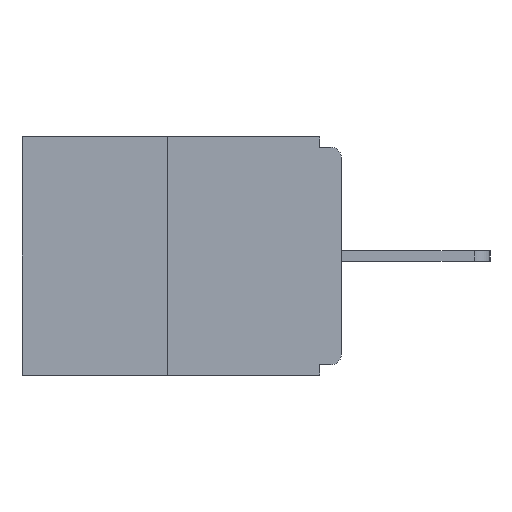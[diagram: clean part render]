
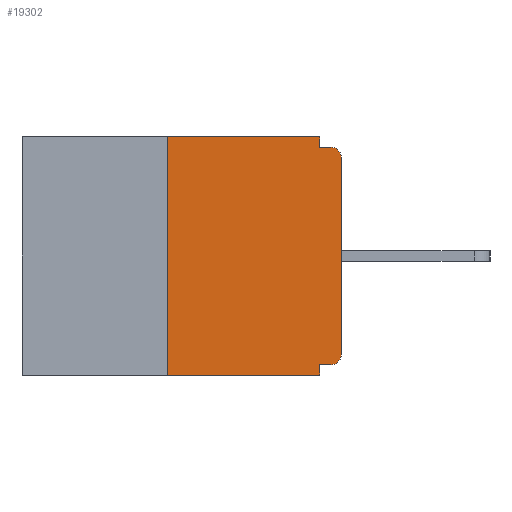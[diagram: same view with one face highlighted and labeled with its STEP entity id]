
A CAD part, left-side view. The second image highlights one B-rep face of the part: STEP entity #19302.
In plain terms, the highlighted planar face has unit normal (-1, 0, 0).
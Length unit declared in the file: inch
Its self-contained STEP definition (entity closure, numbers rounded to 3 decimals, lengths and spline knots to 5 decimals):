
#71 = CIRCLE ( 'NONE', #488, 0.015 ) ;
#295 = CIRCLE ( 'NONE', #757, 0.015 ) ;
#488 = AXIS2_PLACEMENT_3D ( 'NONE', #14695, #5281, #16189 ) ;
#510 = ORIENTED_EDGE ( 'NONE', *, *, #3146, .F. ) ;
#752 = LINE ( 'NONE', #2765, #15977 ) ;
#757 = AXIS2_PLACEMENT_3D ( 'NONE', #793, #11916, #2405 ) ;
#784 = VECTOR ( 'NONE', #14460, 39.37008 ) ;
#793 = CARTESIAN_POINT ( 'NONE',  ( 0., 0.015, -0.03 ) ) ;
#1218 = VERTEX_POINT ( 'NONE', #6164 ) ;
#1501 = CARTESIAN_POINT ( 'NONE',  ( 0., 0.031, 0. ) ) ;
#2095 = CARTESIAN_POINT ( 'NONE',  ( 0., 0.25, 0. ) ) ;
#2405 = DIRECTION ( 'NONE',  ( 0., 0., -1. ) ) ;
#2521 = ORIENTED_EDGE ( 'NONE', *, *, #6641, .T. ) ;
#2597 = CARTESIAN_POINT ( 'NONE',  ( 0., 0.46, 0. ) ) ;
#2736 = VERTEX_POINT ( 'NONE', #19652 ) ;
#2765 = CARTESIAN_POINT ( 'NONE',  ( 0., 0.46, 0. ) ) ;
#3141 = VERTEX_POINT ( 'NONE', #15288 ) ;
#3146 = EDGE_CURVE ( 'NONE', #7224, #12963, #14024, .T. ) ;
#3345 = VERTEX_POINT ( 'NONE', #4631 ) ;
#3429 = DIRECTION ( 'NONE',  ( 0., -1., 0. ) ) ;
#3578 = LINE ( 'NONE', #6592, #8379 ) ;
#3845 = EDGE_LOOP ( 'NONE', ( #17428, #7527, #12204, #510, #9498, #17673, #9998, #2521, #15074, #7292 ) ) ;
#4193 = DIRECTION ( 'NONE',  ( 1., 0., 0. ) ) ;
#4539 = VECTOR ( 'NONE', #6926, 39.37008 ) ;
#4591 = LINE ( 'NONE', #16106, #12038 ) ;
#4631 = CARTESIAN_POINT ( 'NONE',  ( 0., 0.25, 0. ) ) ;
#5037 = CARTESIAN_POINT ( 'NONE',  ( 0., 0., -0.328 ) ) ;
#5263 = DIRECTION ( 'NONE',  ( 0., -1., 0. ) ) ;
#5281 = DIRECTION ( 'NONE',  ( -1., 0., 0. ) ) ;
#5658 = CARTESIAN_POINT ( 'NONE',  ( 0., 0.25, -0.343 ) ) ;
#5968 = EDGE_CURVE ( 'NONE', #1218, #2736, #71, .T. ) ;
#6164 = CARTESIAN_POINT ( 'NONE',  ( 0., 0.015, -0.328 ) ) ;
#6345 = FACE_OUTER_BOUND ( 'NONE', #3845, .T. ) ;
#6592 = CARTESIAN_POINT ( 'NONE',  ( 0., 0.031, 0. ) ) ;
#6641 = EDGE_CURVE ( 'NONE', #3141, #7332, #295, .T. ) ;
#6662 = CARTESIAN_POINT ( 'NONE',  ( 0., 0.46, -0.343 ) ) ;
#6926 = DIRECTION ( 'NONE',  ( 0., 0., 1. ) ) ;
#7074 = EDGE_CURVE ( 'NONE', #1218, #7224, #9294, .T. ) ;
#7218 = CARTESIAN_POINT ( 'NONE',  ( 0., 0.015, -0.015 ) ) ;
#7224 = VERTEX_POINT ( 'NONE', #8549 ) ;
#7292 = ORIENTED_EDGE ( 'NONE', *, *, #11396, .F. ) ;
#7332 = VERTEX_POINT ( 'NONE', #7218 ) ;
#7371 = VECTOR ( 'NONE', #5263, 39.37008 ) ;
#7527 = ORIENTED_EDGE ( 'NONE', *, *, #15026, .F. ) ;
#7837 = LINE ( 'NONE', #6662, #19626 ) ;
#8379 = VECTOR ( 'NONE', #15891, 39.37008 ) ;
#8440 = DIRECTION ( 'NONE',  ( 0., 0., 1. ) ) ;
#8549 = CARTESIAN_POINT ( 'NONE',  ( 0., 0.031, -0.328 ) ) ;
#8950 = PLANE ( 'NONE',  #14837 ) ;
#9294 = LINE ( 'NONE', #5037, #784 ) ;
#9498 = ORIENTED_EDGE ( 'NONE', *, *, #7074, .F. ) ;
#9998 = ORIENTED_EDGE ( 'NONE', *, *, #13305, .T. ) ;
#10769 = DIRECTION ( 'NONE',  ( 0., -1., 0. ) ) ;
#11396 = EDGE_CURVE ( 'NONE', #18134, #19171, #3578, .T. ) ;
#11543 = LINE ( 'NONE', #16168, #7371 ) ;
#11690 = CARTESIAN_POINT ( 'NONE',  ( 0., 0.031, -0.015 ) ) ;
#11916 = DIRECTION ( 'NONE',  ( -1., 0., 0. ) ) ;
#12038 = VECTOR ( 'NONE', #8440, 39.37008 ) ;
#12204 = ORIENTED_EDGE ( 'NONE', *, *, #14379, .T. ) ;
#12473 = LINE ( 'NONE', #2095, #4539 ) ;
#12963 = VERTEX_POINT ( 'NONE', #13821 ) ;
#13305 = EDGE_CURVE ( 'NONE', #2736, #3141, #4591, .T. ) ;
#13336 = EDGE_CURVE ( 'NONE', #19171, #7332, #11543, .T. ) ;
#13821 = CARTESIAN_POINT ( 'NONE',  ( 0., 0.031, -0.343 ) ) ;
#14024 = LINE ( 'NONE', #15166, #17098 ) ;
#14379 = EDGE_CURVE ( 'NONE', #17227, #12963, #7837, .T. ) ;
#14460 = DIRECTION ( 'NONE',  ( 0., 1., 0. ) ) ;
#14695 = CARTESIAN_POINT ( 'NONE',  ( 0., 0.015, -0.313 ) ) ;
#14837 = AXIS2_PLACEMENT_3D ( 'NONE', #2597, #4193, #15189 ) ;
#15026 = EDGE_CURVE ( 'NONE', #17227, #3345, #12473, .T. ) ;
#15074 = ORIENTED_EDGE ( 'NONE', *, *, #13336, .F. ) ;
#15166 = CARTESIAN_POINT ( 'NONE',  ( 0., 0.031, -0.343 ) ) ;
#15189 = DIRECTION ( 'NONE',  ( 0., 0., -1. ) ) ;
#15288 = CARTESIAN_POINT ( 'NONE',  ( 0., 0., -0.03 ) ) ;
#15482 = DIRECTION ( 'NONE',  ( 0., 0., -1. ) ) ;
#15808 = EDGE_CURVE ( 'NONE', #3345, #18134, #752, .T. ) ;
#15891 = DIRECTION ( 'NONE',  ( 0., 0., -1. ) ) ;
#15977 = VECTOR ( 'NONE', #10769, 39.37008 ) ;
#16106 = CARTESIAN_POINT ( 'NONE',  ( 0., 0., 0. ) ) ;
#16168 = CARTESIAN_POINT ( 'NONE',  ( 0., 0., -0.015 ) ) ;
#16189 = DIRECTION ( 'NONE',  ( 0., 0., -1. ) ) ;
#17098 = VECTOR ( 'NONE', #15482, 39.37008 ) ;
#17227 = VERTEX_POINT ( 'NONE', #5658 ) ;
#17428 = ORIENTED_EDGE ( 'NONE', *, *, #15808, .F. ) ;
#17673 = ORIENTED_EDGE ( 'NONE', *, *, #5968, .T. ) ;
#18134 = VERTEX_POINT ( 'NONE', #1501 ) ;
#19171 = VERTEX_POINT ( 'NONE', #11690 ) ;
#19302 = ADVANCED_FACE ( 'NONE', ( #6345 ), #8950, .F. ) ;
#19626 = VECTOR ( 'NONE', #3429, 39.37008 ) ;
#19652 = CARTESIAN_POINT ( 'NONE',  ( 0., 0., -0.313 ) ) ;
